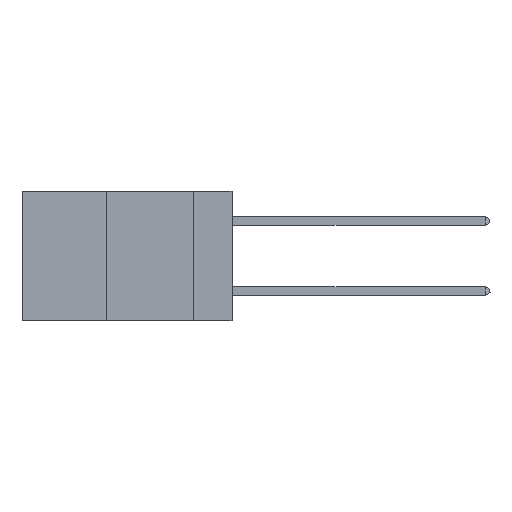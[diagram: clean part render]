
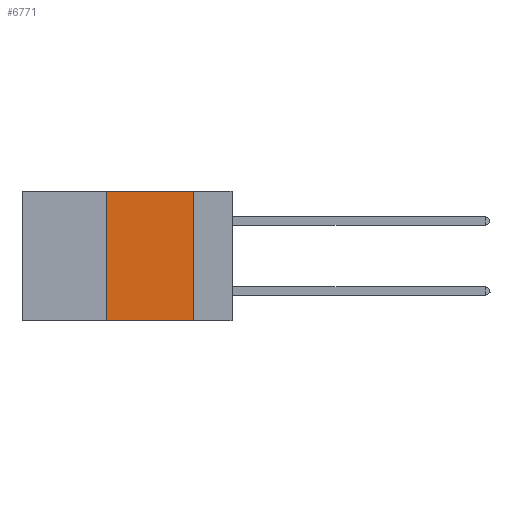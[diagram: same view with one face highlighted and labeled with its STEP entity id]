
A CAD part, left-side view. The second image highlights one B-rep face of the part: STEP entity #6771.
In plain terms, the highlighted planar face has unit normal (-1, 0, 0).
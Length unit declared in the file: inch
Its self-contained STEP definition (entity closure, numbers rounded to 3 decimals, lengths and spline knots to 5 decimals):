
#377 = ORIENTED_EDGE ( 'NONE', *, *, #20879, .F. ) ;
#840 = CARTESIAN_POINT ( 'NONE',  ( 0., 0.6, -0.37 ) ) ;
#1523 = EDGE_CURVE ( 'NONE', #26277, #26953, #7938, .T. ) ;
#2650 = ORIENTED_EDGE ( 'NONE', *, *, #1523, .F. ) ;
#3374 = VERTEX_POINT ( 'NONE', #10114 ) ;
#3500 = FACE_OUTER_BOUND ( 'NONE', #26083, .T. ) ;
#6540 = DIRECTION ( 'NONE',  ( 0., -1., 0. ) ) ;
#6686 = EDGE_CURVE ( 'NONE', #26277, #3374, #19206, .T. ) ;
#6771 = ADVANCED_FACE ( 'NONE', ( #3500 ), #7406, .F. ) ;
#7406 = PLANE ( 'NONE',  #18128 ) ;
#7938 = LINE ( 'NONE', #10664, #19942 ) ;
#8116 = CARTESIAN_POINT ( 'NONE',  ( 0., 0.36, 0. ) ) ;
#9554 = DIRECTION ( 'NONE',  ( 1., 0., 0. ) ) ;
#10114 = CARTESIAN_POINT ( 'NONE',  ( 0., 0.11, -0.37 ) ) ;
#10664 = CARTESIAN_POINT ( 'NONE',  ( 0., 0.36, 0. ) ) ;
#11497 = LINE ( 'NONE', #24726, #12488 ) ;
#12488 = VECTOR ( 'NONE', #20317, 39.37008 ) ;
#13369 = VECTOR ( 'NONE', #6540, 39.37008 ) ;
#13375 = EDGE_CURVE ( 'NONE', #14794, #3374, #11497, .T. ) ;
#14205 = VECTOR ( 'NONE', #22238, 39.37008 ) ;
#14637 = ORIENTED_EDGE ( 'NONE', *, *, #13375, .F. ) ;
#14794 = VERTEX_POINT ( 'NONE', #19873 ) ;
#15900 = CARTESIAN_POINT ( 'NONE',  ( 0., 0.36, -0.37 ) ) ;
#17280 = CARTESIAN_POINT ( 'NONE',  ( 0., 0.6, 0. ) ) ;
#17361 = DIRECTION ( 'NONE',  ( 0., 0., 1. ) ) ;
#18035 = LINE ( 'NONE', #17280, #13369 ) ;
#18128 = AXIS2_PLACEMENT_3D ( 'NONE', #22331, #9554, #24496 ) ;
#19206 = LINE ( 'NONE', #840, #14205 ) ;
#19873 = CARTESIAN_POINT ( 'NONE',  ( 0., 0.11, 0. ) ) ;
#19942 = VECTOR ( 'NONE', #17361, 39.37008 ) ;
#20317 = DIRECTION ( 'NONE',  ( 0., 0., -1. ) ) ;
#20879 = EDGE_CURVE ( 'NONE', #26953, #14794, #18035, .T. ) ;
#22096 = ORIENTED_EDGE ( 'NONE', *, *, #6686, .T. ) ;
#22238 = DIRECTION ( 'NONE',  ( 0., -1., 0. ) ) ;
#22331 = CARTESIAN_POINT ( 'NONE',  ( 0., 0.6, 0. ) ) ;
#24496 = DIRECTION ( 'NONE',  ( 0., 0., -1. ) ) ;
#24726 = CARTESIAN_POINT ( 'NONE',  ( 0., 0.11, 0. ) ) ;
#26083 = EDGE_LOOP ( 'NONE', ( #14637, #377, #2650, #22096 ) ) ;
#26277 = VERTEX_POINT ( 'NONE', #15900 ) ;
#26953 = VERTEX_POINT ( 'NONE', #8116 ) ;
